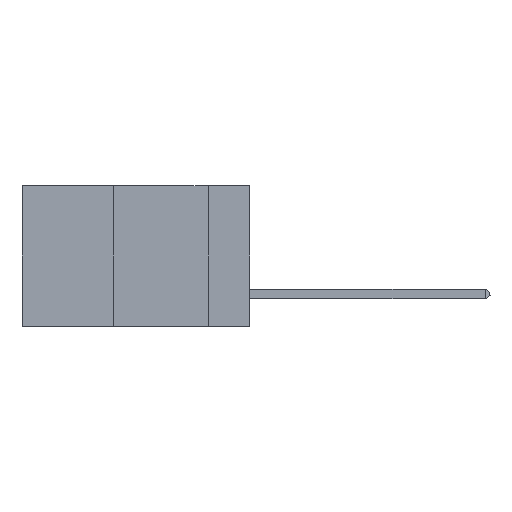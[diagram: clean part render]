
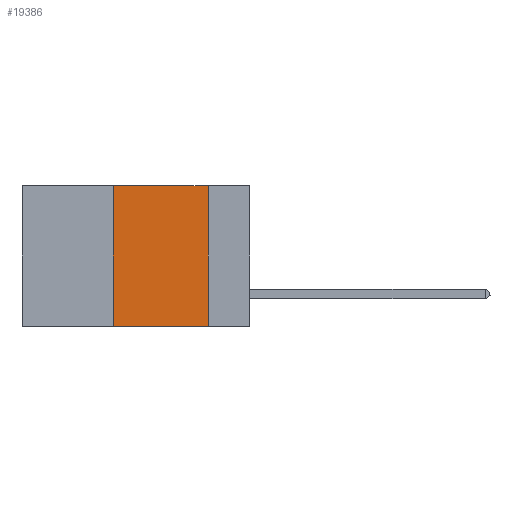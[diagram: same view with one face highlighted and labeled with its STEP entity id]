
A CAD part, left-side view. The second image highlights one B-rep face of the part: STEP entity #19386.
In plain terms, the highlighted planar face has unit normal (-1, 0, 0).
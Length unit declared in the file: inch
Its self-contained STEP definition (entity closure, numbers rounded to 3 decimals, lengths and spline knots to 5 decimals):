
#21 = VERTEX_POINT ( 'NONE', #9996 ) ;
#371 = DIRECTION ( 'NONE',  ( 1., 0., 0. ) ) ;
#945 = CARTESIAN_POINT ( 'NONE',  ( 0., 0.36, 0. ) ) ;
#1328 = CARTESIAN_POINT ( 'NONE',  ( 0., 0.11, 0. ) ) ;
#1343 = PLANE ( 'NONE',  #7840 ) ;
#1980 = VECTOR ( 'NONE', #20048, 39.37008 ) ;
#3325 = EDGE_LOOP ( 'NONE', ( #12115, #6582, #19505, #5603 ) ) ;
#5603 = ORIENTED_EDGE ( 'NONE', *, *, #24239, .T. ) ;
#5673 = VERTEX_POINT ( 'NONE', #945 ) ;
#5875 = VECTOR ( 'NONE', #22716, 39.37008 ) ;
#6249 = LINE ( 'NONE', #16806, #14044 ) ;
#6582 = ORIENTED_EDGE ( 'NONE', *, *, #7321, .F. ) ;
#7321 = EDGE_CURVE ( 'NONE', #5673, #14496, #23696, .T. ) ;
#7544 = CARTESIAN_POINT ( 'NONE',  ( 0., 0.6, -0.37 ) ) ;
#7840 = AXIS2_PLACEMENT_3D ( 'NONE', #23186, #371, #19903 ) ;
#9996 = CARTESIAN_POINT ( 'NONE',  ( 0., 0.11, -0.37 ) ) ;
#10606 = VERTEX_POINT ( 'NONE', #24826 ) ;
#11481 = LINE ( 'NONE', #1328, #12079 ) ;
#12079 = VECTOR ( 'NONE', #13018, 39.37008 ) ;
#12115 = ORIENTED_EDGE ( 'NONE', *, *, #20408, .F. ) ;
#13018 = DIRECTION ( 'NONE',  ( 0., 0., -1. ) ) ;
#13316 = EDGE_CURVE ( 'NONE', #10606, #5673, #6249, .T. ) ;
#14044 = VECTOR ( 'NONE', #18578, 39.37008 ) ;
#14175 = CARTESIAN_POINT ( 'NONE',  ( 0., 0.6, 0. ) ) ;
#14496 = VERTEX_POINT ( 'NONE', #17974 ) ;
#14989 = FACE_OUTER_BOUND ( 'NONE', #3325, .T. ) ;
#16806 = CARTESIAN_POINT ( 'NONE',  ( 0., 0.36, 0. ) ) ;
#17974 = CARTESIAN_POINT ( 'NONE',  ( 0., 0.11, 0. ) ) ;
#18578 = DIRECTION ( 'NONE',  ( 0., 0., 1. ) ) ;
#18844 = LINE ( 'NONE', #7544, #5875 ) ;
#19386 = ADVANCED_FACE ( 'NONE', ( #14989 ), #1343, .F. ) ;
#19505 = ORIENTED_EDGE ( 'NONE', *, *, #13316, .F. ) ;
#19903 = DIRECTION ( 'NONE',  ( 0., 0., -1. ) ) ;
#20048 = DIRECTION ( 'NONE',  ( 0., -1., 0. ) ) ;
#20408 = EDGE_CURVE ( 'NONE', #14496, #21, #11481, .T. ) ;
#22716 = DIRECTION ( 'NONE',  ( 0., -1., 0. ) ) ;
#23186 = CARTESIAN_POINT ( 'NONE',  ( 0., 0.6, 0. ) ) ;
#23696 = LINE ( 'NONE', #14175, #1980 ) ;
#24239 = EDGE_CURVE ( 'NONE', #10606, #21, #18844, .T. ) ;
#24826 = CARTESIAN_POINT ( 'NONE',  ( 0., 0.36, -0.37 ) ) ;
